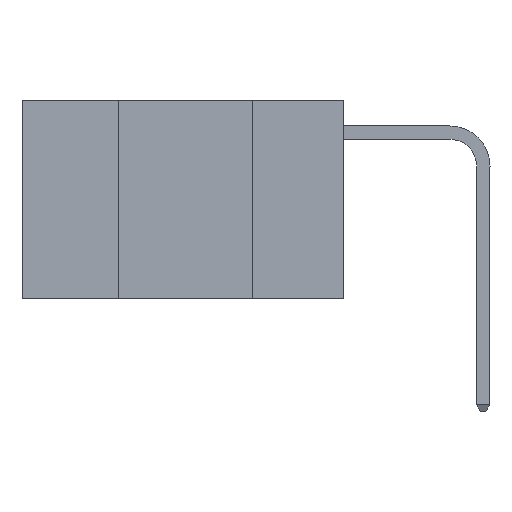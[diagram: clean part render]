
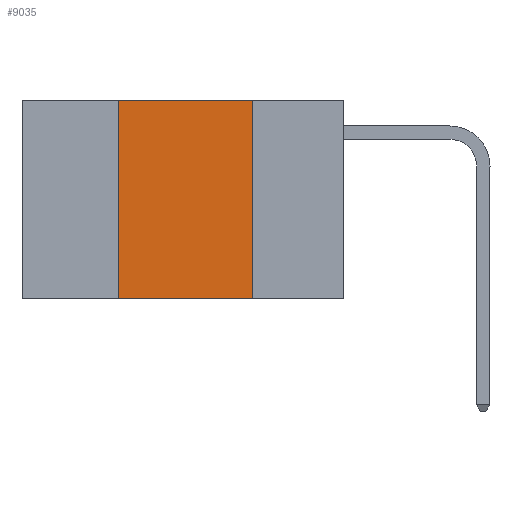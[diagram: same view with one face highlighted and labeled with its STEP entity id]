
A CAD part, left-side view. The second image highlights one B-rep face of the part: STEP entity #9035.
In plain terms, the highlighted planar face has unit normal (-1, 0, 0).
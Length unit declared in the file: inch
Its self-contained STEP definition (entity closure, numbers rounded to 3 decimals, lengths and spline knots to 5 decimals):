
#240 = VERTEX_POINT ( 'NONE', #11661 ) ;
#1380 = CARTESIAN_POINT ( 'NONE',  ( 0., 0.17, 0. ) ) ;
#1744 = VECTOR ( 'NONE', #9281, 39.37008 ) ;
#2036 = LINE ( 'NONE', #12669, #1744 ) ;
#2286 = DIRECTION ( 'NONE',  ( 0., 0., -1. ) ) ;
#2738 = EDGE_CURVE ( 'NONE', #13075, #14711, #2036, .T. ) ;
#2751 = VECTOR ( 'NONE', #5229, 39.37008 ) ;
#2855 = LINE ( 'NONE', #12315, #2751 ) ;
#3061 = DIRECTION ( 'NONE',  ( 0., 0., -1. ) ) ;
#3134 = CARTESIAN_POINT ( 'NONE',  ( 0., 0.42, -0.37 ) ) ;
#4898 = LINE ( 'NONE', #11901, #13823 ) ;
#5215 = CARTESIAN_POINT ( 'NONE',  ( 0., 0.42, 0. ) ) ;
#5229 = DIRECTION ( 'NONE',  ( 0., 0., 1. ) ) ;
#5488 = VERTEX_POINT ( 'NONE', #3134 ) ;
#5979 = DIRECTION ( 'NONE',  ( 0., -1., 0. ) ) ;
#7597 = ORIENTED_EDGE ( 'NONE', *, *, #13415, .F. ) ;
#7842 = ORIENTED_EDGE ( 'NONE', *, *, #2738, .F. ) ;
#7855 = ORIENTED_EDGE ( 'NONE', *, *, #9600, .F. ) ;
#7943 = ORIENTED_EDGE ( 'NONE', *, *, #10396, .T. ) ;
#8957 = CARTESIAN_POINT ( 'NONE',  ( 0., 0.6, 0. ) ) ;
#9000 = PLANE ( 'NONE',  #14850 ) ;
#9035 = ADVANCED_FACE ( 'NONE', ( #11088 ), #9000, .F. ) ;
#9281 = DIRECTION ( 'NONE',  ( 0., -1., 0. ) ) ;
#9600 = EDGE_CURVE ( 'NONE', #5488, #13075, #2855, .T. ) ;
#10196 = DIRECTION ( 'NONE',  ( 1., 0., 0. ) ) ;
#10396 = EDGE_CURVE ( 'NONE', #5488, #240, #4898, .T. ) ;
#10951 = LINE ( 'NONE', #12860, #13243 ) ;
#11088 = FACE_OUTER_BOUND ( 'NONE', #11844, .T. ) ;
#11661 = CARTESIAN_POINT ( 'NONE',  ( 0., 0.17, -0.37 ) ) ;
#11844 = EDGE_LOOP ( 'NONE', ( #7597, #7842, #7855, #7943 ) ) ;
#11901 = CARTESIAN_POINT ( 'NONE',  ( 0., 0.6, -0.37 ) ) ;
#12315 = CARTESIAN_POINT ( 'NONE',  ( 0., 0.42, 0. ) ) ;
#12669 = CARTESIAN_POINT ( 'NONE',  ( 0., 0.6, 0. ) ) ;
#12860 = CARTESIAN_POINT ( 'NONE',  ( 0., 0.17, 0. ) ) ;
#13075 = VERTEX_POINT ( 'NONE', #5215 ) ;
#13243 = VECTOR ( 'NONE', #2286, 39.37008 ) ;
#13415 = EDGE_CURVE ( 'NONE', #14711, #240, #10951, .T. ) ;
#13823 = VECTOR ( 'NONE', #5979, 39.37008 ) ;
#14711 = VERTEX_POINT ( 'NONE', #1380 ) ;
#14850 = AXIS2_PLACEMENT_3D ( 'NONE', #8957, #10196, #3061 ) ;
